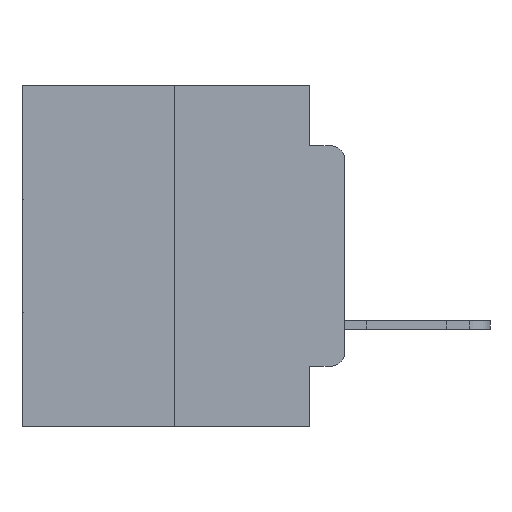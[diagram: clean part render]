
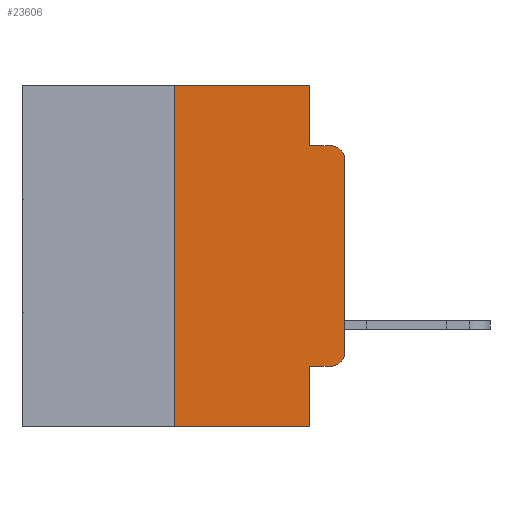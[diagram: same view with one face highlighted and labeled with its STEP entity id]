
A CAD part, left-side view. The second image highlights one B-rep face of the part: STEP entity #23606.
In plain terms, the highlighted planar face has unit normal (-1, 0, 0).
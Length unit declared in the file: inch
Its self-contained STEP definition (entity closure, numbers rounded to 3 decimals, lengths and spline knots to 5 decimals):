
#251 = LINE ( 'NONE', #21242, #9190 ) ;
#976 = EDGE_CURVE ( 'NONE', #18481, #21472, #251, .T. ) ;
#1408 = ORIENTED_EDGE ( 'NONE', *, *, #9081, .T. ) ;
#1478 = CARTESIAN_POINT ( 'NONE',  ( 0., 0.051, 0. ) ) ;
#1703 = VERTEX_POINT ( 'NONE', #8883 ) ;
#1739 = AXIS2_PLACEMENT_3D ( 'NONE', #25227, #21002, #12093 ) ;
#2537 = CARTESIAN_POINT ( 'NONE',  ( 0., 0.051, -0.0885 ) ) ;
#2829 = EDGE_CURVE ( 'NONE', #7099, #16129, #11482, .T. ) ;
#3634 = VECTOR ( 'NONE', #20113, 39.37008 ) ;
#3715 = ORIENTED_EDGE ( 'NONE', *, *, #2829, .F. ) ;
#4632 = CARTESIAN_POINT ( 'NONE',  ( 0., 0.02, -0.1085 ) ) ;
#4789 = VECTOR ( 'NONE', #27628, 39.37008 ) ;
#5012 = EDGE_CURVE ( 'NONE', #10219, #7099, #8893, .T. ) ;
#5612 = EDGE_LOOP ( 'NONE', ( #5770, #13133, #20008, #3715, #18808, #26309, #15637, #26000, #9234, #1408 ) ) ;
#5770 = ORIENTED_EDGE ( 'NONE', *, *, #976, .T. ) ;
#5843 = AXIS2_PLACEMENT_3D ( 'NONE', #4632, #6565, #11037 ) ;
#6280 = CARTESIAN_POINT ( 'NONE',  ( 0., 0.051, -0.4115 ) ) ;
#6565 = DIRECTION ( 'NONE',  ( -1., 0., 0. ) ) ;
#6718 = EDGE_CURVE ( 'NONE', #10932, #10219, #16352, .T. ) ;
#6927 = FACE_OUTER_BOUND ( 'NONE', #5612, .T. ) ;
#7099 = VERTEX_POINT ( 'NONE', #12565 ) ;
#7140 = VERTEX_POINT ( 'NONE', #6280 ) ;
#7240 = EDGE_CURVE ( 'NONE', #21472, #20200, #19394, .T. ) ;
#8648 = CARTESIAN_POINT ( 'NONE',  ( 0., 0.051, 0. ) ) ;
#8883 = CARTESIAN_POINT ( 'NONE',  ( 0., 0.02, -0.4115 ) ) ;
#8893 = LINE ( 'NONE', #12711, #9930 ) ;
#9081 = EDGE_CURVE ( 'NONE', #1703, #18481, #12415, .T. ) ;
#9190 = VECTOR ( 'NONE', #25636, 39.37008 ) ;
#9234 = ORIENTED_EDGE ( 'NONE', *, *, #21604, .T. ) ;
#9334 = LINE ( 'NONE', #8648, #12759 ) ;
#9481 = CARTESIAN_POINT ( 'NONE',  ( 0., 0.02, -0.0885 ) ) ;
#9843 = VERTEX_POINT ( 'NONE', #20899 ) ;
#9930 = VECTOR ( 'NONE', #13064, 39.37008 ) ;
#10219 = VERTEX_POINT ( 'NONE', #19265 ) ;
#10609 = LINE ( 'NONE', #27908, #4789 ) ;
#10932 = VERTEX_POINT ( 'NONE', #25938 ) ;
#11037 = DIRECTION ( 'NONE',  ( 0., 0., -1. ) ) ;
#11482 = LINE ( 'NONE', #1478, #21776 ) ;
#11907 = LINE ( 'NONE', #15220, #15664 ) ;
#12093 = DIRECTION ( 'NONE',  ( 0., 0., -1. ) ) ;
#12415 = CIRCLE ( 'NONE', #26619, 0.02 ) ;
#12565 = CARTESIAN_POINT ( 'NONE',  ( 0., 0.051, 0. ) ) ;
#12711 = CARTESIAN_POINT ( 'NONE',  ( 0., 0.473, 0. ) ) ;
#12759 = VECTOR ( 'NONE', #26353, 39.37008 ) ;
#13064 = DIRECTION ( 'NONE',  ( 0., -1., 0. ) ) ;
#13133 = ORIENTED_EDGE ( 'NONE', *, *, #7240, .T. ) ;
#13175 = DIRECTION ( 'NONE',  ( 0., -1., 0. ) ) ;
#13481 = CARTESIAN_POINT ( 'NONE',  ( 0., 0.25, 0. ) ) ;
#13661 = EDGE_CURVE ( 'NONE', #10932, #9843, #11907, .T. ) ;
#14083 = CARTESIAN_POINT ( 'NONE',  ( 0., 0., -0.3915 ) ) ;
#15220 = CARTESIAN_POINT ( 'NONE',  ( 0., 0.473, -0.5 ) ) ;
#15637 = ORIENTED_EDGE ( 'NONE', *, *, #13661, .T. ) ;
#15664 = VECTOR ( 'NONE', #13175, 39.37008 ) ;
#16129 = VERTEX_POINT ( 'NONE', #2537 ) ;
#16352 = LINE ( 'NONE', #13481, #3634 ) ;
#18481 = VERTEX_POINT ( 'NONE', #14083 ) ;
#18589 = PLANE ( 'NONE',  #1739 ) ;
#18808 = ORIENTED_EDGE ( 'NONE', *, *, #5012, .F. ) ;
#19265 = CARTESIAN_POINT ( 'NONE',  ( 0., 0.25, 0. ) ) ;
#19394 = CIRCLE ( 'NONE', #5843, 0.02 ) ;
#19662 = CARTESIAN_POINT ( 'NONE',  ( 0., 0.051, -0.0885 ) ) ;
#19941 = EDGE_CURVE ( 'NONE', #7140, #9843, #9334, .T. ) ;
#20008 = ORIENTED_EDGE ( 'NONE', *, *, #23113, .F. ) ;
#20113 = DIRECTION ( 'NONE',  ( 0., 0., 1. ) ) ;
#20200 = VERTEX_POINT ( 'NONE', #9481 ) ;
#20623 = CARTESIAN_POINT ( 'NONE',  ( 0., 0., -0.1085 ) ) ;
#20899 = CARTESIAN_POINT ( 'NONE',  ( 0., 0.051, -0.5 ) ) ;
#21002 = DIRECTION ( 'NONE',  ( 1., 0., 0. ) ) ;
#21242 = CARTESIAN_POINT ( 'NONE',  ( 0., 0., 0. ) ) ;
#21472 = VERTEX_POINT ( 'NONE', #20623 ) ;
#21604 = EDGE_CURVE ( 'NONE', #7140, #1703, #10609, .T. ) ;
#21703 = DIRECTION ( 'NONE',  ( 0., -1., 0. ) ) ;
#21776 = VECTOR ( 'NONE', #25256, 39.37008 ) ;
#23113 = EDGE_CURVE ( 'NONE', #16129, #20200, #23720, .T. ) ;
#23606 = ADVANCED_FACE ( 'NONE', ( #6927 ), #18589, .F. ) ;
#23720 = LINE ( 'NONE', #19662, #25761 ) ;
#24007 = DIRECTION ( 'NONE',  ( 0., 0., -1. ) ) ;
#25227 = CARTESIAN_POINT ( 'NONE',  ( 0., 0.473, 0. ) ) ;
#25256 = DIRECTION ( 'NONE',  ( 0., 0., -1. ) ) ;
#25523 = CARTESIAN_POINT ( 'NONE',  ( 0., 0.02, -0.3915 ) ) ;
#25636 = DIRECTION ( 'NONE',  ( 0., 0., 1. ) ) ;
#25761 = VECTOR ( 'NONE', #21703, 39.37008 ) ;
#25938 = CARTESIAN_POINT ( 'NONE',  ( 0., 0.25, -0.5 ) ) ;
#26000 = ORIENTED_EDGE ( 'NONE', *, *, #19941, .F. ) ;
#26309 = ORIENTED_EDGE ( 'NONE', *, *, #6718, .F. ) ;
#26353 = DIRECTION ( 'NONE',  ( 0., 0., -1. ) ) ;
#26619 = AXIS2_PLACEMENT_3D ( 'NONE', #25523, #27822, #24007 ) ;
#27628 = DIRECTION ( 'NONE',  ( 0., -1., 0. ) ) ;
#27822 = DIRECTION ( 'NONE',  ( -1., 0., 0. ) ) ;
#27908 = CARTESIAN_POINT ( 'NONE',  ( 0., 0.051, -0.4115 ) ) ;
